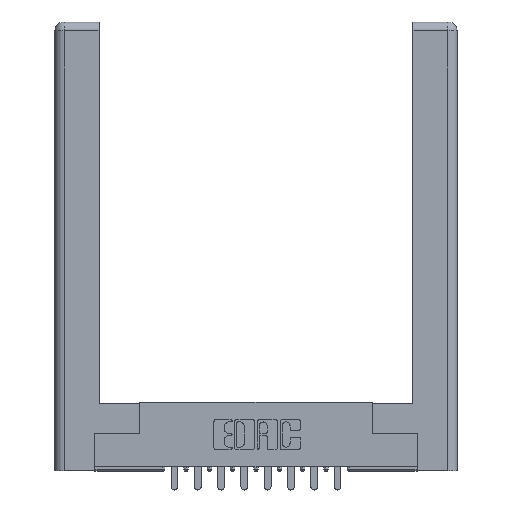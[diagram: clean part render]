
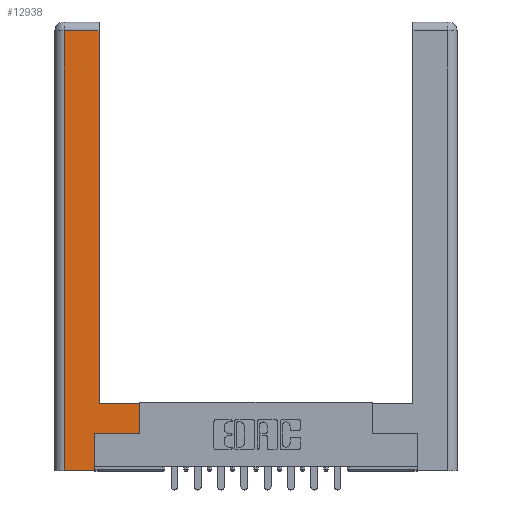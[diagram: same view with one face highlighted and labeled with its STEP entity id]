
A CAD part, top view. The second image highlights one B-rep face of the part: STEP entity #12938.
In plain terms, the highlighted planar face has unit normal (0, 0, 1).
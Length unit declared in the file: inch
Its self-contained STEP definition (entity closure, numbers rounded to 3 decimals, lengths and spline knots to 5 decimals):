
#223 = CARTESIAN_POINT ( 'NONE',  ( 0.565, 0.45, 0. ) ) ;
#255 = DIRECTION ( 'NONE',  ( 0., 1., 0. ) ) ;
#300 = CARTESIAN_POINT ( 'NONE',  ( 0.0615, 0., 0. ) ) ;
#604 = DIRECTION ( 'NONE',  ( 0., -1., 0. ) ) ;
#820 = CARTESIAN_POINT ( 'NONE',  ( 0.565, 0.245, 0. ) ) ;
#960 = VERTEX_POINT ( 'NONE', #300 ) ;
#1023 = CARTESIAN_POINT ( 'NONE',  ( 0.265, 0.245, 0. ) ) ;
#1324 = VERTEX_POINT ( 'NONE', #14054 ) ;
#1829 = LINE ( 'NONE', #13454, #2953 ) ;
#2013 = DIRECTION ( 'NONE',  ( 1., 0., 0. ) ) ;
#2051 = VERTEX_POINT ( 'NONE', #223 ) ;
#2160 = EDGE_CURVE ( 'NONE', #960, #9560, #4867, .T. ) ;
#2228 = EDGE_CURVE ( 'NONE', #3551, #2051, #4325, .T. ) ;
#2315 = EDGE_CURVE ( 'NONE', #9560, #8539, #10600, .T. ) ;
#2399 = CARTESIAN_POINT ( 'NONE',  ( 0.295, 0.45, 0. ) ) ;
#2897 = DIRECTION ( 'NONE',  ( -1., 0., 0. ) ) ;
#2953 = VECTOR ( 'NONE', #5279, 39.37008 ) ;
#3087 = CARTESIAN_POINT ( 'NONE',  ( 0.0615, 0., 0. ) ) ;
#3430 = CARTESIAN_POINT ( 'NONE',  ( 0.295, 0.45, 0. ) ) ;
#3551 = VERTEX_POINT ( 'NONE', #12384 ) ;
#3626 = ORIENTED_EDGE ( 'NONE', *, *, #12232, .T. ) ;
#3687 = VECTOR ( 'NONE', #15182, 39.37008 ) ;
#3860 = CARTESIAN_POINT ( 'NONE',  ( 0.295, 2.94, 0. ) ) ;
#3958 = VECTOR ( 'NONE', #13469, 39.37008 ) ;
#4019 = DIRECTION ( 'NONE',  ( 1., 0., 0. ) ) ;
#4325 = LINE ( 'NONE', #11106, #3958 ) ;
#4867 = LINE ( 'NONE', #14526, #9523 ) ;
#5244 = DIRECTION ( 'NONE',  ( 0., 0., -1. ) ) ;
#5279 = DIRECTION ( 'NONE',  ( -1., 0., 0. ) ) ;
#5422 = VECTOR ( 'NONE', #14686, 39.37008 ) ;
#5488 = EDGE_CURVE ( 'NONE', #2051, #13188, #5876, .T. ) ;
#5876 = LINE ( 'NONE', #3430, #3687 ) ;
#6829 = EDGE_CURVE ( 'NONE', #13188, #8078, #9571, .T. ) ;
#6988 = ORIENTED_EDGE ( 'NONE', *, *, #2315, .T. ) ;
#7382 = EDGE_LOOP ( 'NONE', ( #11985, #9622, #3626, #8591, #6988, #9580, #14324, #14366 ) ) ;
#8078 = VERTEX_POINT ( 'NONE', #3860 ) ;
#8539 = VERTEX_POINT ( 'NONE', #1023 ) ;
#8591 = ORIENTED_EDGE ( 'NONE', *, *, #2160, .T. ) ;
#8763 = EDGE_CURVE ( 'NONE', #8078, #1324, #1829, .T. ) ;
#8867 = CARTESIAN_POINT ( 'NONE',  ( 0., 0., 0. ) ) ;
#9132 = FACE_OUTER_BOUND ( 'NONE', #7382, .T. ) ;
#9260 = VECTOR ( 'NONE', #2013, 39.37008 ) ;
#9523 = VECTOR ( 'NONE', #4019, 39.37008 ) ;
#9560 = VERTEX_POINT ( 'NONE', #14435 ) ;
#9571 = LINE ( 'NONE', #13094, #14891 ) ;
#9580 = ORIENTED_EDGE ( 'NONE', *, *, #15114, .T. ) ;
#9622 = ORIENTED_EDGE ( 'NONE', *, *, #8763, .T. ) ;
#9668 = AXIS2_PLACEMENT_3D ( 'NONE', #8867, #5244, #2897 ) ;
#10074 = PLANE ( 'NONE',  #9668 ) ;
#10600 = LINE ( 'NONE', #12434, #5422 ) ;
#11106 = CARTESIAN_POINT ( 'NONE',  ( 0.565, 0.45, 0. ) ) ;
#11985 = ORIENTED_EDGE ( 'NONE', *, *, #6829, .T. ) ;
#12232 = EDGE_CURVE ( 'NONE', #1324, #960, #12811, .T. ) ;
#12281 = VECTOR ( 'NONE', #604, 39.37008 ) ;
#12384 = CARTESIAN_POINT ( 'NONE',  ( 0.565, 0.245, 0. ) ) ;
#12434 = CARTESIAN_POINT ( 'NONE',  ( 0.265, 0.245, 0. ) ) ;
#12811 = LINE ( 'NONE', #3087, #12281 ) ;
#12938 = ADVANCED_FACE ( 'NONE', ( #9132 ), #10074, .F. ) ;
#13094 = CARTESIAN_POINT ( 'NONE',  ( 0.295, 3., 0. ) ) ;
#13188 = VERTEX_POINT ( 'NONE', #2399 ) ;
#13454 = CARTESIAN_POINT ( 'NONE',  ( 0.0615, 2.94, 0. ) ) ;
#13469 = DIRECTION ( 'NONE',  ( 0., 1., 0. ) ) ;
#14054 = CARTESIAN_POINT ( 'NONE',  ( 0.0615, 2.94, 0. ) ) ;
#14324 = ORIENTED_EDGE ( 'NONE', *, *, #2228, .T. ) ;
#14365 = LINE ( 'NONE', #820, #9260 ) ;
#14366 = ORIENTED_EDGE ( 'NONE', *, *, #5488, .T. ) ;
#14435 = CARTESIAN_POINT ( 'NONE',  ( 0.265, 0., 0. ) ) ;
#14526 = CARTESIAN_POINT ( 'NONE',  ( 0.265, 0., 0. ) ) ;
#14686 = DIRECTION ( 'NONE',  ( 0., 1., 0. ) ) ;
#14891 = VECTOR ( 'NONE', #255, 39.37008 ) ;
#15114 = EDGE_CURVE ( 'NONE', #8539, #3551, #14365, .T. ) ;
#15182 = DIRECTION ( 'NONE',  ( -1., 0., 0. ) ) ;
